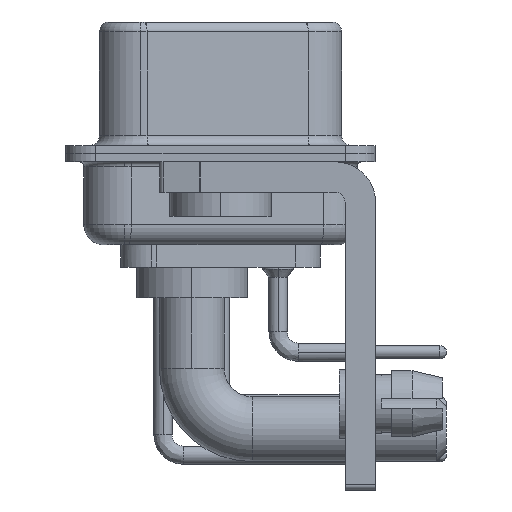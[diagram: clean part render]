
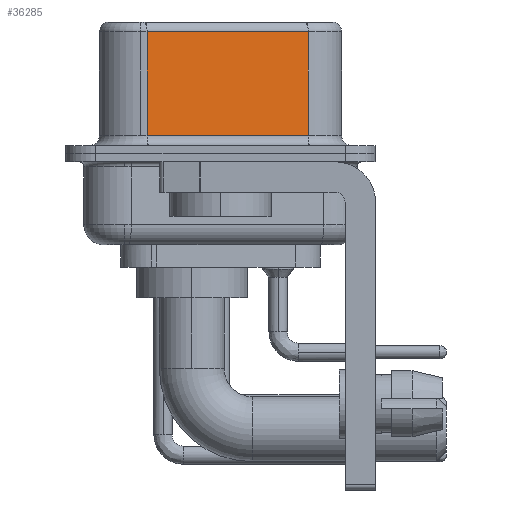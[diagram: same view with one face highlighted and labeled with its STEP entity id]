
A CAD part, left-side view. The second image highlights one B-rep face of the part: STEP entity #36285.
In plain terms, the highlighted planar face has unit normal (-0.985, -0.174, 0).
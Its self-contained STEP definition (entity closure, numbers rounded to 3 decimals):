
#1801 = DIRECTION ( 'NONE',  ( 0., 0., -1. ) ) ;
#2167 = PLANE ( 'NONE',  #8932 ) ;
#2430 = ORIENTED_EDGE ( 'NONE', *, *, #19630, .T. ) ;
#5773 = VECTOR ( 'NONE', #12127, 1000. ) ;
#6837 = DIRECTION ( 'NONE',  ( -0.174, 0.985, 0. ) ) ;
#7937 = ORIENTED_EDGE ( 'NONE', *, *, #8626, .T. ) ;
#8381 = ORIENTED_EDGE ( 'NONE', *, *, #34728, .F. ) ;
#8626 = EDGE_CURVE ( 'NONE', #10062, #29249, #26826, .T. ) ;
#8932 = AXIS2_PLACEMENT_3D ( 'NONE', #11091, #10908, #19469 ) ;
#10062 = VERTEX_POINT ( 'NONE', #18128 ) ;
#10617 = VECTOR ( 'NONE', #1801, 1000. ) ;
#10908 = DIRECTION ( 'NONE',  ( 0.985, 0.174, 0. ) ) ;
#11091 = CARTESIAN_POINT ( 'NONE',  ( 5.132, -4.322, 6.52 ) ) ;
#11441 = CARTESIAN_POINT ( 'NONE',  ( 5.132, -4.322, 6.52 ) ) ;
#11643 = VECTOR ( 'NONE', #6837, 1000. ) ;
#12127 = DIRECTION ( 'NONE',  ( 0.174, -0.985, 0. ) ) ;
#12841 = VERTEX_POINT ( 'NONE', #28845 ) ;
#13602 = EDGE_LOOP ( 'NONE', ( #8381, #22171, #2430, #7937 ) ) ;
#17776 = VECTOR ( 'NONE', #31718, 1000. ) ;
#18012 = CARTESIAN_POINT ( 'NONE',  ( 5.132, -4.322, 6.02 ) ) ;
#18128 = CARTESIAN_POINT ( 'NONE',  ( 3.73, 3.628, 0.9 ) ) ;
#19469 = DIRECTION ( 'NONE',  ( -0.174, 0.985, 0. ) ) ;
#19630 = EDGE_CURVE ( 'NONE', #29418, #10062, #21342, .T. ) ;
#20834 = CARTESIAN_POINT ( 'NONE',  ( 3.73, 3.628, 6.02 ) ) ;
#21342 = LINE ( 'NONE', #24150, #10617 ) ;
#22171 = ORIENTED_EDGE ( 'NONE', *, *, #31185, .T. ) ;
#24150 = CARTESIAN_POINT ( 'NONE',  ( 3.73, 3.628, 6.52 ) ) ;
#25967 = LINE ( 'NONE', #11441, #17776 ) ;
#26826 = LINE ( 'NONE', #32408, #5773 ) ;
#28845 = CARTESIAN_POINT ( 'NONE',  ( 5.132, -4.322, 6.02 ) ) ;
#29249 = VERTEX_POINT ( 'NONE', #34784 ) ;
#29418 = VERTEX_POINT ( 'NONE', #20834 ) ;
#30811 = FACE_OUTER_BOUND ( 'NONE', #13602, .T. ) ;
#31185 = EDGE_CURVE ( 'NONE', #12841, #29418, #32515, .T. ) ;
#31718 = DIRECTION ( 'NONE',  ( 0., 0., -1. ) ) ;
#32408 = CARTESIAN_POINT ( 'NONE',  ( 5.132, -4.322, 0.9 ) ) ;
#32515 = LINE ( 'NONE', #18012, #11643 ) ;
#34728 = EDGE_CURVE ( 'NONE', #12841, #29249, #25967, .T. ) ;
#34784 = CARTESIAN_POINT ( 'NONE',  ( 5.132, -4.322, 0.9 ) ) ;
#36285 = ADVANCED_FACE ( 'NONE', ( #30811 ), #2167, .F. ) ;
